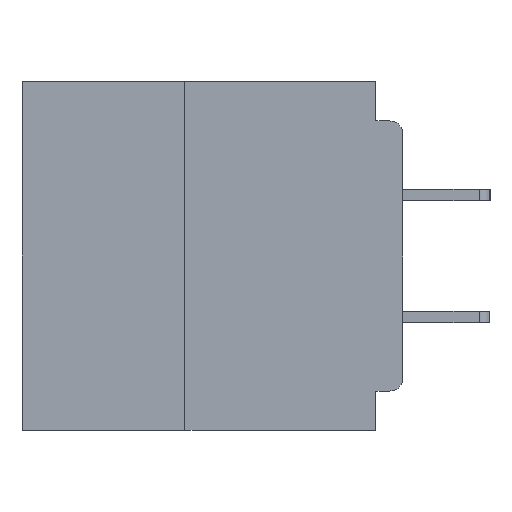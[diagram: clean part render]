
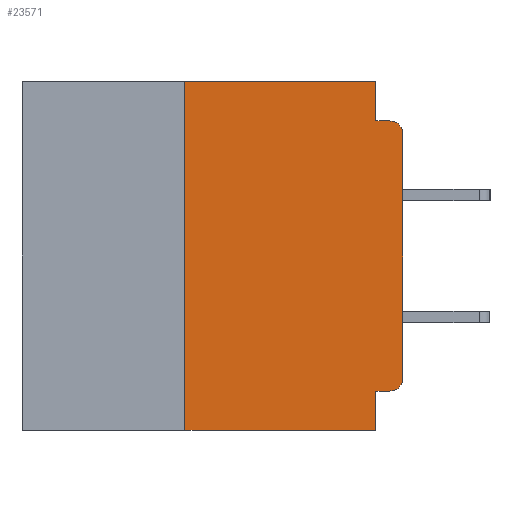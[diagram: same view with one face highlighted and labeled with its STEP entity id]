
A CAD part, left-side view. The second image highlights one B-rep face of the part: STEP entity #23571.
In plain terms, the highlighted planar face has unit normal (-1, 0, 0).
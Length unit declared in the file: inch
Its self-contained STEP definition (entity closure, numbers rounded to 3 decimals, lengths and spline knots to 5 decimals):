
#772 = DIRECTION ( 'NONE',  ( -1., 0., 0. ) ) ;
#791 = VECTOR ( 'NONE', #846, 39.37008 ) ;
#846 = DIRECTION ( 'NONE',  ( 0., -1., 0. ) ) ;
#2490 = CARTESIAN_POINT ( 'NONE',  ( 0., 0.031, -0.355 ) ) ;
#3218 = CARTESIAN_POINT ( 'NONE',  ( 0., 0.437, 0. ) ) ;
#3270 = DIRECTION ( 'NONE',  ( 0., 0., -1. ) ) ;
#4411 = LINE ( 'NONE', #47320, #43517 ) ;
#4476 = CARTESIAN_POINT ( 'NONE',  ( 0., 0.25, 0. ) ) ;
#4550 = CARTESIAN_POINT ( 'NONE',  ( 0., 0.437, -0.4 ) ) ;
#5366 = VERTEX_POINT ( 'NONE', #46153 ) ;
#6496 = EDGE_CURVE ( 'NONE', #19204, #23098, #6773, .T. ) ;
#6773 = LINE ( 'NONE', #30619, #35879 ) ;
#6778 = ORIENTED_EDGE ( 'NONE', *, *, #44528, .F. ) ;
#7813 = CARTESIAN_POINT ( 'NONE',  ( 0., 0.031, -0.045 ) ) ;
#7937 = EDGE_CURVE ( 'NONE', #15682, #39976, #10805, .T. ) ;
#8311 = LINE ( 'NONE', #14522, #35006 ) ;
#9906 = CARTESIAN_POINT ( 'NONE',  ( 0., 0.015, -0.06 ) ) ;
#10805 = LINE ( 'NONE', #31894, #48642 ) ;
#10843 = AXIS2_PLACEMENT_3D ( 'NONE', #23587, #772, #27429 ) ;
#10971 = ORIENTED_EDGE ( 'NONE', *, *, #31739, .F. ) ;
#12200 = ORIENTED_EDGE ( 'NONE', *, *, #6496, .F. ) ;
#13513 = CARTESIAN_POINT ( 'NONE',  ( 0., 0.015, -0.045 ) ) ;
#13521 = DIRECTION ( 'NONE',  ( 0., 0., -1. ) ) ;
#13719 = DIRECTION ( 'NONE',  ( 0., 0., -1. ) ) ;
#14522 = CARTESIAN_POINT ( 'NONE',  ( 0., 0.031, -0.4 ) ) ;
#14575 = PLANE ( 'NONE',  #42712 ) ;
#14918 = ORIENTED_EDGE ( 'NONE', *, *, #26531, .T. ) ;
#15682 = VERTEX_POINT ( 'NONE', #28697 ) ;
#15782 = ORIENTED_EDGE ( 'NONE', *, *, #33900, .F. ) ;
#16448 = FACE_OUTER_BOUND ( 'NONE', #32558, .T. ) ;
#16633 = VERTEX_POINT ( 'NONE', #35019 ) ;
#17454 = ORIENTED_EDGE ( 'NONE', *, *, #37142, .F. ) ;
#18526 = DIRECTION ( 'NONE',  ( 0., 0., -1. ) ) ;
#19095 = CARTESIAN_POINT ( 'NONE',  ( 0., 0.25, -0.4 ) ) ;
#19204 = VERTEX_POINT ( 'NONE', #19095 ) ;
#19407 = LINE ( 'NONE', #4550, #48336 ) ;
#19969 = EDGE_CURVE ( 'NONE', #19204, #31254, #19407, .T. ) ;
#20784 = LINE ( 'NONE', #3218, #48523 ) ;
#21039 = ORIENTED_EDGE ( 'NONE', *, *, #7937, .T. ) ;
#21059 = LINE ( 'NONE', #27499, #791 ) ;
#21616 = ORIENTED_EDGE ( 'NONE', *, *, #48512, .F. ) ;
#22955 = DIRECTION ( 'NONE',  ( 0., 0., 1. ) ) ;
#23032 = VERTEX_POINT ( 'NONE', #7813 ) ;
#23098 = VERTEX_POINT ( 'NONE', #4476 ) ;
#23225 = CARTESIAN_POINT ( 'NONE',  ( 0., 0.031, -0.4 ) ) ;
#23571 = ADVANCED_FACE ( 'NONE', ( #16448 ), #14575, .F. ) ;
#23587 = CARTESIAN_POINT ( 'NONE',  ( 0., 0.015, -0.34 ) ) ;
#24749 = DIRECTION ( 'NONE',  ( 0., 1., 0. ) ) ;
#26068 = DIRECTION ( 'NONE',  ( 1., 0., 0. ) ) ;
#26531 = EDGE_CURVE ( 'NONE', #5366, #15682, #41645, .T. ) ;
#27352 = DIRECTION ( 'NONE',  ( 0., -1., 0. ) ) ;
#27429 = DIRECTION ( 'NONE',  ( 0., 0., -1. ) ) ;
#27499 = CARTESIAN_POINT ( 'NONE',  ( 0., 0., -0.045 ) ) ;
#28697 = CARTESIAN_POINT ( 'NONE',  ( 0., 0., -0.34 ) ) ;
#29825 = DIRECTION ( 'NONE',  ( 0., -1., 0. ) ) ;
#30150 = LINE ( 'NONE', #47573, #48953 ) ;
#30441 = VERTEX_POINT ( 'NONE', #2490 ) ;
#30619 = CARTESIAN_POINT ( 'NONE',  ( 0., 0.25, -0.4 ) ) ;
#31254 = VERTEX_POINT ( 'NONE', #23225 ) ;
#31739 = EDGE_CURVE ( 'NONE', #23098, #16633, #20784, .T. ) ;
#31894 = CARTESIAN_POINT ( 'NONE',  ( 0., 0., 0. ) ) ;
#32246 = DIRECTION ( 'NONE',  ( 0., 0., 1. ) ) ;
#32558 = EDGE_LOOP ( 'NONE', ( #21039, #44108, #17454, #15782, #10971, #12200, #41888, #21616, #6778, #14918 ) ) ;
#33900 = EDGE_CURVE ( 'NONE', #16633, #23032, #30150, .T. ) ;
#34102 = AXIS2_PLACEMENT_3D ( 'NONE', #9906, #36428, #13719 ) ;
#34566 = CIRCLE ( 'NONE', #34102, 0.015 ) ;
#35006 = VECTOR ( 'NONE', #18526, 39.37008 ) ;
#35019 = CARTESIAN_POINT ( 'NONE',  ( 0., 0.031, 0. ) ) ;
#35868 = VERTEX_POINT ( 'NONE', #13513 ) ;
#35879 = VECTOR ( 'NONE', #22955, 39.37008 ) ;
#36428 = DIRECTION ( 'NONE',  ( -1., 0., 0. ) ) ;
#37142 = EDGE_CURVE ( 'NONE', #23032, #35868, #21059, .T. ) ;
#38325 = CARTESIAN_POINT ( 'NONE',  ( 0., 0., -0.06 ) ) ;
#39976 = VERTEX_POINT ( 'NONE', #38325 ) ;
#41645 = CIRCLE ( 'NONE', #10843, 0.015 ) ;
#41888 = ORIENTED_EDGE ( 'NONE', *, *, #19969, .T. ) ;
#42712 = AXIS2_PLACEMENT_3D ( 'NONE', #48611, #26068, #3270 ) ;
#43517 = VECTOR ( 'NONE', #24749, 39.37008 ) ;
#44108 = ORIENTED_EDGE ( 'NONE', *, *, #45839, .T. ) ;
#44528 = EDGE_CURVE ( 'NONE', #5366, #30441, #4411, .T. ) ;
#45839 = EDGE_CURVE ( 'NONE', #39976, #35868, #34566, .T. ) ;
#46153 = CARTESIAN_POINT ( 'NONE',  ( 0., 0.015, -0.355 ) ) ;
#47320 = CARTESIAN_POINT ( 'NONE',  ( 0., 0., -0.355 ) ) ;
#47573 = CARTESIAN_POINT ( 'NONE',  ( 0., 0.031, 0. ) ) ;
#48336 = VECTOR ( 'NONE', #27352, 39.37008 ) ;
#48512 = EDGE_CURVE ( 'NONE', #30441, #31254, #8311, .T. ) ;
#48523 = VECTOR ( 'NONE', #29825, 39.37008 ) ;
#48611 = CARTESIAN_POINT ( 'NONE',  ( 0., 0.437, 0. ) ) ;
#48642 = VECTOR ( 'NONE', #32246, 39.37008 ) ;
#48953 = VECTOR ( 'NONE', #13521, 39.37008 ) ;
